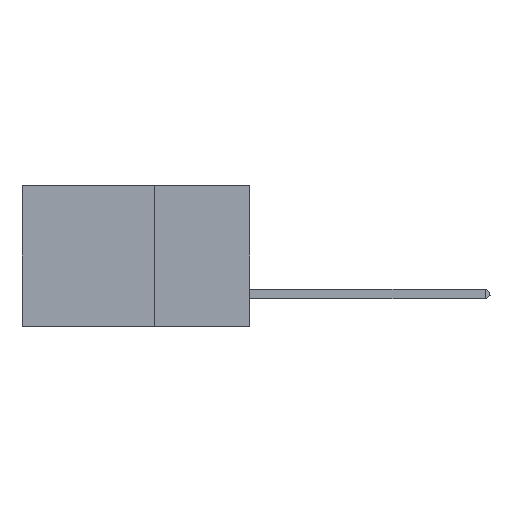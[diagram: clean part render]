
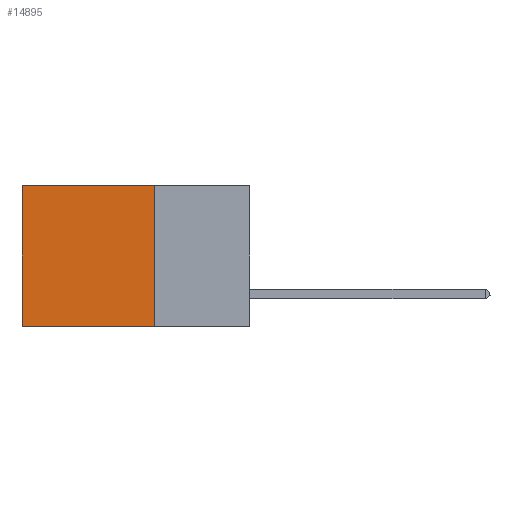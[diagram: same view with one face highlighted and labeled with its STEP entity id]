
A CAD part, left-side view. The second image highlights one B-rep face of the part: STEP entity #14895.
In plain terms, the highlighted planar face has unit normal (-1, 0, 0).
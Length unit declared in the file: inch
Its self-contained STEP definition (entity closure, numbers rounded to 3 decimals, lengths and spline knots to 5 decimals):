
#122 = VECTOR ( 'NONE', #12460, 39.37008 ) ;
#456 = CARTESIAN_POINT ( 'NONE',  ( 0.2875, 0.25, -0.37 ) ) ;
#968 = VERTEX_POINT ( 'NONE', #15972 ) ;
#1028 = CARTESIAN_POINT ( 'NONE',  ( 0.2875, 0.25, 0. ) ) ;
#1536 = LINE ( 'NONE', #13416, #14632 ) ;
#2500 = VECTOR ( 'NONE', #7063, 39.37008 ) ;
#4593 = PLANE ( 'NONE',  #6004 ) ;
#5244 = EDGE_CURVE ( 'NONE', #13888, #6355, #13449, .T. ) ;
#5731 = EDGE_CURVE ( 'NONE', #968, #11656, #6241, .T. ) ;
#6004 = AXIS2_PLACEMENT_3D ( 'NONE', #1028, #12296, #14801 ) ;
#6241 = LINE ( 'NONE', #15048, #9126 ) ;
#6355 = VERTEX_POINT ( 'NONE', #456 ) ;
#6607 = CARTESIAN_POINT ( 'NONE',  ( 0.2875, 0.6, -0.37 ) ) ;
#6945 = ORIENTED_EDGE ( 'NONE', *, *, #15559, .F. ) ;
#7063 = DIRECTION ( 'NONE',  ( 0., 0., -1. ) ) ;
#7129 = ORIENTED_EDGE ( 'NONE', *, *, #11835, .T. ) ;
#8409 = FACE_OUTER_BOUND ( 'NONE', #11213, .T. ) ;
#9126 = VECTOR ( 'NONE', #12476, 39.37008 ) ;
#9482 = CARTESIAN_POINT ( 'NONE',  ( 0.2875, 0.25, 0. ) ) ;
#10965 = DIRECTION ( 'NONE',  ( 0., 1., 0. ) ) ;
#11213 = EDGE_LOOP ( 'NONE', ( #15062, #6945, #13743, #7129 ) ) ;
#11656 = VERTEX_POINT ( 'NONE', #6607 ) ;
#11835 = EDGE_CURVE ( 'NONE', #13888, #968, #12434, .T. ) ;
#12296 = DIRECTION ( 'NONE',  ( 1., 0., 0. ) ) ;
#12434 = LINE ( 'NONE', #12576, #122 ) ;
#12460 = DIRECTION ( 'NONE',  ( 0., 1., 0. ) ) ;
#12476 = DIRECTION ( 'NONE',  ( 0., 0., -1. ) ) ;
#12576 = CARTESIAN_POINT ( 'NONE',  ( 0.2875, 0.25, 0. ) ) ;
#13416 = CARTESIAN_POINT ( 'NONE',  ( 0.2875, 0.25, -0.37 ) ) ;
#13449 = LINE ( 'NONE', #9482, #2500 ) ;
#13743 = ORIENTED_EDGE ( 'NONE', *, *, #5244, .F. ) ;
#13888 = VERTEX_POINT ( 'NONE', #15772 ) ;
#14632 = VECTOR ( 'NONE', #10965, 39.37008 ) ;
#14801 = DIRECTION ( 'NONE',  ( 0., 0., -1. ) ) ;
#14895 = ADVANCED_FACE ( 'NONE', ( #8409 ), #4593, .F. ) ;
#15048 = CARTESIAN_POINT ( 'NONE',  ( 0.2875, 0.6, 0. ) ) ;
#15062 = ORIENTED_EDGE ( 'NONE', *, *, #5731, .T. ) ;
#15559 = EDGE_CURVE ( 'NONE', #6355, #11656, #1536, .T. ) ;
#15772 = CARTESIAN_POINT ( 'NONE',  ( 0.2875, 0.25, 0. ) ) ;
#15972 = CARTESIAN_POINT ( 'NONE',  ( 0.2875, 0.6, 0. ) ) ;
